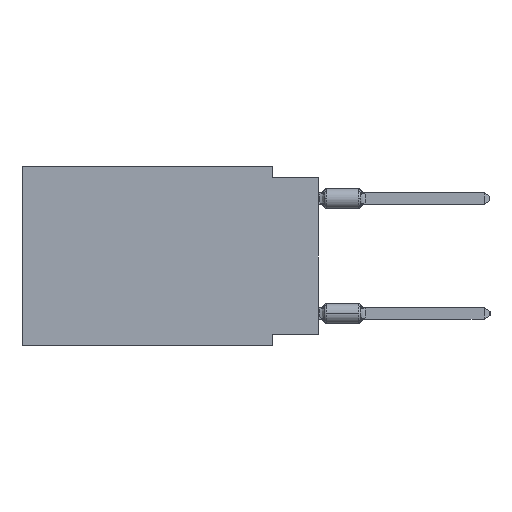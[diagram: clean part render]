
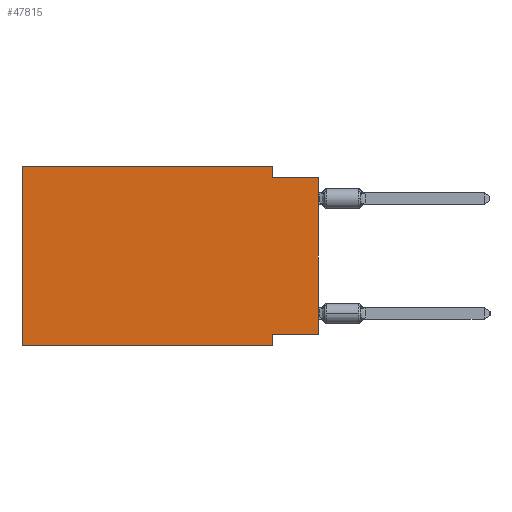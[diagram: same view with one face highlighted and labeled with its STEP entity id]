
A CAD part, left-side view. The second image highlights one B-rep face of the part: STEP entity #47815.
In plain terms, the highlighted planar face has unit normal (-1, 0, 0).
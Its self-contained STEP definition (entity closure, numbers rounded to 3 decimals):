
#1025 = DIRECTION ( 'NONE',  ( 0., 0., 1. ) ) ;
#1087 = CARTESIAN_POINT ( 'NONE',  ( 0., 16.383, -9.906 ) ) ;
#1488 = LINE ( 'NONE', #31988, #8015 ) ;
#1495 = ORIENTED_EDGE ( 'NONE', *, *, #19002, .F. ) ;
#1747 = LINE ( 'NONE', #16485, #23244 ) ;
#1760 = AXIS2_PLACEMENT_3D ( 'NONE', #1834, #43309, #27802 ) ;
#1834 = CARTESIAN_POINT ( 'NONE',  ( 0., 16.383, 0. ) ) ;
#3425 = VECTOR ( 'NONE', #42435, 1000. ) ;
#4200 = LINE ( 'NONE', #22443, #3425 ) ;
#5032 = EDGE_CURVE ( 'NONE', #23711, #37516, #47357, .T. ) ;
#6641 = CARTESIAN_POINT ( 'NONE',  ( 0., 2.54, 0. ) ) ;
#7811 = CARTESIAN_POINT ( 'NONE',  ( 0., 0., -9.271 ) ) ;
#8015 = VECTOR ( 'NONE', #1025, 1000. ) ;
#8477 = ORIENTED_EDGE ( 'NONE', *, *, #42547, .F. ) ;
#9315 = VERTEX_POINT ( 'NONE', #1087 ) ;
#11252 = ORIENTED_EDGE ( 'NONE', *, *, #24769, .T. ) ;
#16479 = DIRECTION ( 'NONE',  ( 0., 0., -1. ) ) ;
#16485 = CARTESIAN_POINT ( 'NONE',  ( 0., 16.383, -9.906 ) ) ;
#16929 = CARTESIAN_POINT ( 'NONE',  ( 0., 2.54, -0.635 ) ) ;
#17194 = ORIENTED_EDGE ( 'NONE', *, *, #5032, .F. ) ;
#17387 = DIRECTION ( 'NONE',  ( 0., -1., 0. ) ) ;
#17809 = EDGE_LOOP ( 'NONE', ( #46399, #1495, #8477, #17194, #44134, #11252, #28792, #41399 ) ) ;
#19002 = EDGE_CURVE ( 'NONE', #19540, #25708, #32902, .T. ) ;
#19169 = VECTOR ( 'NONE', #16479, 1000. ) ;
#19540 = VERTEX_POINT ( 'NONE', #16929 ) ;
#19572 = VERTEX_POINT ( 'NONE', #32172 ) ;
#21372 = EDGE_CURVE ( 'NONE', #47495, #19572, #26802, .T. ) ;
#22169 = VECTOR ( 'NONE', #25339, 1000. ) ;
#22443 = CARTESIAN_POINT ( 'NONE',  ( 0., 16.383, 0. ) ) ;
#23244 = VECTOR ( 'NONE', #23968, 1000. ) ;
#23711 = VERTEX_POINT ( 'NONE', #30356 ) ;
#23968 = DIRECTION ( 'NONE',  ( 0., -1., 0. ) ) ;
#24227 = LINE ( 'NONE', #31229, #19169 ) ;
#24769 = EDGE_CURVE ( 'NONE', #9315, #36755, #1747, .T. ) ;
#25141 = CARTESIAN_POINT ( 'NONE',  ( 0., 0., -0.635 ) ) ;
#25339 = DIRECTION ( 'NONE',  ( 0., -1., 0. ) ) ;
#25607 = LINE ( 'NONE', #6641, #49404 ) ;
#25708 = VERTEX_POINT ( 'NONE', #28772 ) ;
#26089 = DIRECTION ( 'NONE',  ( 0., 0., -1. ) ) ;
#26802 = LINE ( 'NONE', #7811, #42597 ) ;
#27628 = EDGE_CURVE ( 'NONE', #47495, #25708, #1488, .T. ) ;
#27802 = DIRECTION ( 'NONE',  ( 0., 0., -1. ) ) ;
#28772 = CARTESIAN_POINT ( 'NONE',  ( 0., 0., -0.635 ) ) ;
#28792 = ORIENTED_EDGE ( 'NONE', *, *, #31645, .F. ) ;
#30356 = CARTESIAN_POINT ( 'NONE',  ( 0., 16.383, 0. ) ) ;
#31186 = CARTESIAN_POINT ( 'NONE',  ( 0., 0., -9.271 ) ) ;
#31229 = CARTESIAN_POINT ( 'NONE',  ( 0., 2.54, -9.906 ) ) ;
#31645 = EDGE_CURVE ( 'NONE', #19572, #36755, #24227, .T. ) ;
#31988 = CARTESIAN_POINT ( 'NONE',  ( 0., 0., 0. ) ) ;
#32172 = CARTESIAN_POINT ( 'NONE',  ( 0., 2.54, -9.271 ) ) ;
#32902 = LINE ( 'NONE', #25141, #43354 ) ;
#35848 = CARTESIAN_POINT ( 'NONE',  ( 0., 16.383, 0. ) ) ;
#36755 = VERTEX_POINT ( 'NONE', #45104 ) ;
#37516 = VERTEX_POINT ( 'NONE', #45668 ) ;
#38806 = FACE_OUTER_BOUND ( 'NONE', #17809, .T. ) ;
#39308 = EDGE_CURVE ( 'NONE', #9315, #23711, #4200, .T. ) ;
#41399 = ORIENTED_EDGE ( 'NONE', *, *, #21372, .F. ) ;
#42435 = DIRECTION ( 'NONE',  ( 0., 0., 1. ) ) ;
#42547 = EDGE_CURVE ( 'NONE', #37516, #19540, #25607, .T. ) ;
#42597 = VECTOR ( 'NONE', #46040, 1000. ) ;
#43309 = DIRECTION ( 'NONE',  ( 1., 0., 0. ) ) ;
#43354 = VECTOR ( 'NONE', #17387, 1000. ) ;
#44134 = ORIENTED_EDGE ( 'NONE', *, *, #39308, .F. ) ;
#45104 = CARTESIAN_POINT ( 'NONE',  ( 0., 2.54, -9.906 ) ) ;
#45668 = CARTESIAN_POINT ( 'NONE',  ( 0., 2.54, 0. ) ) ;
#46040 = DIRECTION ( 'NONE',  ( 0., 1., 0. ) ) ;
#46399 = ORIENTED_EDGE ( 'NONE', *, *, #27628, .T. ) ;
#47299 = PLANE ( 'NONE',  #1760 ) ;
#47357 = LINE ( 'NONE', #35848, #22169 ) ;
#47495 = VERTEX_POINT ( 'NONE', #31186 ) ;
#47815 = ADVANCED_FACE ( 'NONE', ( #38806 ), #47299, .F. ) ;
#49404 = VECTOR ( 'NONE', #26089, 1000. ) ;
